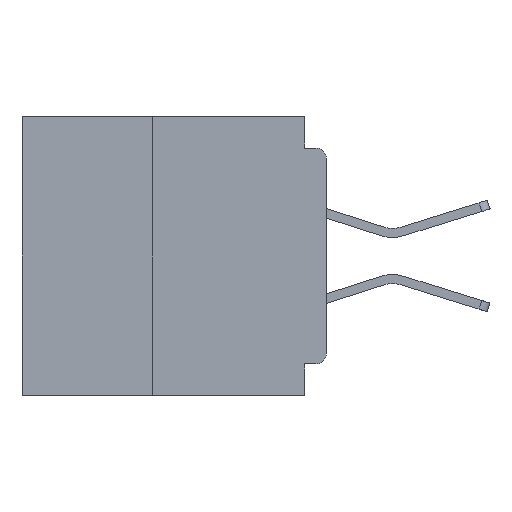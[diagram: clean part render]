
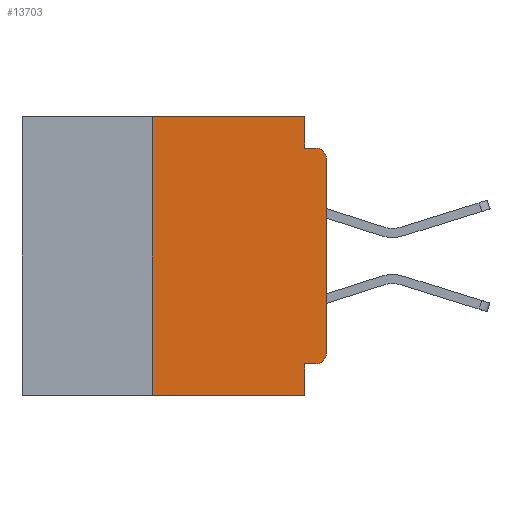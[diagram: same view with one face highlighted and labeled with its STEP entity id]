
A CAD part, left-side view. The second image highlights one B-rep face of the part: STEP entity #13703.
In plain terms, the highlighted planar face has unit normal (-1, 0, 0).
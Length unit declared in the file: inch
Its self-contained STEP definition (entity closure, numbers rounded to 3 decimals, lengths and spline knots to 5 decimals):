
#646 = CARTESIAN_POINT ( 'NONE',  ( 0., 0.015, -0.06 ) ) ;
#1155 = DIRECTION ( 'NONE',  ( 0., 0., -1. ) ) ;
#1313 = DIRECTION ( 'NONE',  ( 0., 0., -1. ) ) ;
#2578 = ORIENTED_EDGE ( 'NONE', *, *, #44689, .F. ) ;
#2838 = CARTESIAN_POINT ( 'NONE',  ( 0., 0., -0.06 ) ) ;
#3840 = EDGE_CURVE ( 'NONE', #48720, #5430, #36942, .T. ) ;
#3846 = AXIS2_PLACEMENT_3D ( 'NONE', #646, #28985, #4704 ) ;
#4080 = VECTOR ( 'NONE', #21392, 39.37008 ) ;
#4704 = DIRECTION ( 'NONE',  ( 0., 0., -1. ) ) ;
#5430 = VERTEX_POINT ( 'NONE', #43040 ) ;
#6651 = ORIENTED_EDGE ( 'NONE', *, *, #11187, .F. ) ;
#7649 = CARTESIAN_POINT ( 'NONE',  ( 0., 0.25, -0.4 ) ) ;
#8681 = CARTESIAN_POINT ( 'NONE',  ( 0., 0.437, -0.4 ) ) ;
#9269 = PLANE ( 'NONE',  #27196 ) ;
#9442 = ORIENTED_EDGE ( 'NONE', *, *, #47299, .F. ) ;
#9583 = ORIENTED_EDGE ( 'NONE', *, *, #14067, .F. ) ;
#10375 = ORIENTED_EDGE ( 'NONE', *, *, #3840, .T. ) ;
#11187 = EDGE_CURVE ( 'NONE', #31266, #5430, #13583, .T. ) ;
#11503 = CIRCLE ( 'NONE', #37719, 0.015 ) ;
#12850 = ORIENTED_EDGE ( 'NONE', *, *, #27956, .T. ) ;
#13129 = CARTESIAN_POINT ( 'NONE',  ( 0., 0.25, -0.4 ) ) ;
#13400 = FACE_OUTER_BOUND ( 'NONE', #33318, .T. ) ;
#13583 = LINE ( 'NONE', #49382, #4080 ) ;
#13703 = ADVANCED_FACE ( 'NONE', ( #13400 ), #9269, .F. ) ;
#14067 = EDGE_CURVE ( 'NONE', #48720, #39331, #34791, .T. ) ;
#14092 = CARTESIAN_POINT ( 'NONE',  ( 0., 0.031, -0.045 ) ) ;
#15021 = CARTESIAN_POINT ( 'NONE',  ( 0., 0., -0.34 ) ) ;
#17012 = EDGE_CURVE ( 'NONE', #17680, #29953, #36865, .T. ) ;
#17452 = CARTESIAN_POINT ( 'NONE',  ( 0., 0.437, 0. ) ) ;
#17454 = DIRECTION ( 'NONE',  ( 0., 0., 1. ) ) ;
#17680 = VERTEX_POINT ( 'NONE', #45618 ) ;
#19009 = CARTESIAN_POINT ( 'NONE',  ( 0., 0.015, -0.045 ) ) ;
#19890 = ORIENTED_EDGE ( 'NONE', *, *, #49901, .T. ) ;
#19901 = DIRECTION ( 'NONE',  ( 0., 0., 1. ) ) ;
#20283 = VECTOR ( 'NONE', #36722, 39.37008 ) ;
#21392 = DIRECTION ( 'NONE',  ( 0., 0., -1. ) ) ;
#21542 = CARTESIAN_POINT ( 'NONE',  ( 0., 0., -0.045 ) ) ;
#22968 = CARTESIAN_POINT ( 'NONE',  ( 0., 0.015, -0.355 ) ) ;
#23571 = VECTOR ( 'NONE', #43935, 39.37008 ) ;
#23983 = VERTEX_POINT ( 'NONE', #2838 ) ;
#24835 = LINE ( 'NONE', #39937, #23571 ) ;
#25472 = DIRECTION ( 'NONE',  ( -1., 0., 0. ) ) ;
#25600 = VERTEX_POINT ( 'NONE', #22968 ) ;
#25630 = DIRECTION ( 'NONE',  ( 1., 0., 0. ) ) ;
#26077 = LINE ( 'NONE', #21542, #36674 ) ;
#26349 = VECTOR ( 'NONE', #44932, 39.37008 ) ;
#27196 = AXIS2_PLACEMENT_3D ( 'NONE', #17452, #25630, #1313 ) ;
#27283 = EDGE_CURVE ( 'NONE', #29953, #50798, #26077, .T. ) ;
#27615 = VERTEX_POINT ( 'NONE', #15021 ) ;
#27956 = EDGE_CURVE ( 'NONE', #25600, #27615, #11503, .T. ) ;
#28985 = DIRECTION ( 'NONE',  ( -1., 0., 0. ) ) ;
#29953 = VERTEX_POINT ( 'NONE', #14092 ) ;
#30065 = ORIENTED_EDGE ( 'NONE', *, *, #17012, .F. ) ;
#31266 = VERTEX_POINT ( 'NONE', #42071 ) ;
#31568 = LINE ( 'NONE', #40564, #20283 ) ;
#32041 = CARTESIAN_POINT ( 'NONE',  ( 0., 0.25, 0. ) ) ;
#33318 = EDGE_LOOP ( 'NONE', ( #19890, #40308, #44547, #30065, #2578, #9583, #10375, #6651, #9442, #12850 ) ) ;
#33497 = CARTESIAN_POINT ( 'NONE',  ( 0., 0., 0. ) ) ;
#33549 = VECTOR ( 'NONE', #19901, 39.37008 ) ;
#34791 = LINE ( 'NONE', #7649, #33549 ) ;
#34801 = CIRCLE ( 'NONE', #3846, 0.015 ) ;
#35604 = VECTOR ( 'NONE', #48813, 39.37008 ) ;
#36674 = VECTOR ( 'NONE', #37617, 39.37008 ) ;
#36722 = DIRECTION ( 'NONE',  ( 0., 1., 0. ) ) ;
#36865 = LINE ( 'NONE', #44795, #35604 ) ;
#36942 = LINE ( 'NONE', #8681, #26349 ) ;
#37617 = DIRECTION ( 'NONE',  ( 0., -1., 0. ) ) ;
#37719 = AXIS2_PLACEMENT_3D ( 'NONE', #49383, #25472, #1155 ) ;
#39331 = VERTEX_POINT ( 'NONE', #32041 ) ;
#39937 = CARTESIAN_POINT ( 'NONE',  ( 0., 0.437, 0. ) ) ;
#40308 = ORIENTED_EDGE ( 'NONE', *, *, #46167, .T. ) ;
#40564 = CARTESIAN_POINT ( 'NONE',  ( 0., 0., -0.355 ) ) ;
#42071 = CARTESIAN_POINT ( 'NONE',  ( 0., 0.031, -0.355 ) ) ;
#43040 = CARTESIAN_POINT ( 'NONE',  ( 0., 0.031, -0.4 ) ) ;
#43803 = VECTOR ( 'NONE', #17454, 39.37008 ) ;
#43935 = DIRECTION ( 'NONE',  ( 0., -1., 0. ) ) ;
#44547 = ORIENTED_EDGE ( 'NONE', *, *, #27283, .F. ) ;
#44689 = EDGE_CURVE ( 'NONE', #39331, #17680, #24835, .T. ) ;
#44795 = CARTESIAN_POINT ( 'NONE',  ( 0., 0.031, 0. ) ) ;
#44932 = DIRECTION ( 'NONE',  ( 0., -1., 0. ) ) ;
#45618 = CARTESIAN_POINT ( 'NONE',  ( 0., 0.031, 0. ) ) ;
#46167 = EDGE_CURVE ( 'NONE', #23983, #50798, #34801, .T. ) ;
#47299 = EDGE_CURVE ( 'NONE', #25600, #31266, #31568, .T. ) ;
#48720 = VERTEX_POINT ( 'NONE', #13129 ) ;
#48813 = DIRECTION ( 'NONE',  ( 0., 0., -1. ) ) ;
#48838 = LINE ( 'NONE', #33497, #43803 ) ;
#49382 = CARTESIAN_POINT ( 'NONE',  ( 0., 0.031, -0.4 ) ) ;
#49383 = CARTESIAN_POINT ( 'NONE',  ( 0., 0.015, -0.34 ) ) ;
#49901 = EDGE_CURVE ( 'NONE', #27615, #23983, #48838, .T. ) ;
#50798 = VERTEX_POINT ( 'NONE', #19009 ) ;
